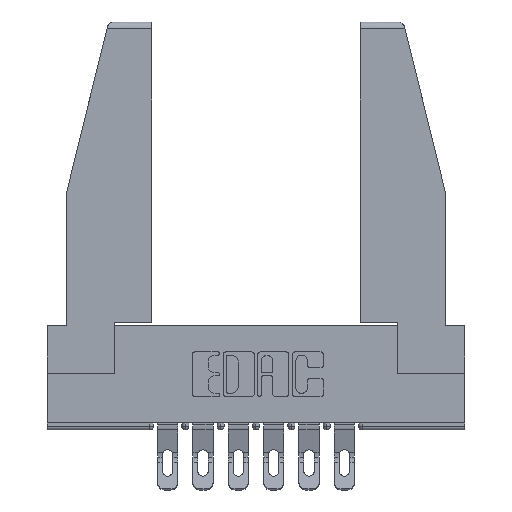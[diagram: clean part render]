
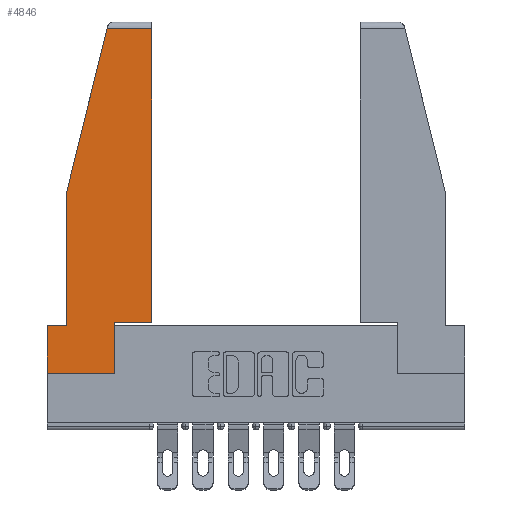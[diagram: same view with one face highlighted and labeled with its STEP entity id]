
A CAD part, top view. The second image highlights one B-rep face of the part: STEP entity #4846.
In plain terms, the highlighted planar face has unit normal (0, 0, 1).
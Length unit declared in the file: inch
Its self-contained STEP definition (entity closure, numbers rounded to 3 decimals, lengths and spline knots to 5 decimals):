
#361 = EDGE_CURVE ( 'NONE', #10906, #6399, #10309, .T. ) ;
#398 = CARTESIAN_POINT ( 'NONE',  ( 0.297, 0.223, 0. ) ) ;
#401 = EDGE_CURVE ( 'NONE', #5165, #10906, #4209, .T. ) ;
#894 = VERTEX_POINT ( 'NONE', #1363 ) ;
#895 = ORIENTED_EDGE ( 'NONE', *, *, #5038, .T. ) ;
#1025 = VECTOR ( 'NONE', #11948, 39.37008 ) ;
#1055 = VECTOR ( 'NONE', #4365, 39.37008 ) ;
#1147 = LINE ( 'NONE', #11577, #8379 ) ;
#1281 = ORIENTED_EDGE ( 'NONE', *, *, #6685, .T. ) ;
#1363 = CARTESIAN_POINT ( 'NONE',  ( 0.461, 0.223, 0. ) ) ;
#1478 = CARTESIAN_POINT ( 'NONE',  ( 0., 0., 0. ) ) ;
#1511 = CARTESIAN_POINT ( 'NONE',  ( 0.461, 0.223, 0. ) ) ;
#1646 = VECTOR ( 'NONE', #2559, 39.37008 ) ;
#1691 = ORIENTED_EDGE ( 'NONE', *, *, #6602, .T. ) ;
#1863 = CARTESIAN_POINT ( 'NONE',  ( 0., 0.21, 0. ) ) ;
#2161 = CARTESIAN_POINT ( 'NONE',  ( 0.461, 1.52, 0. ) ) ;
#2559 = DIRECTION ( 'NONE',  ( 1., 0., 0. ) ) ;
#2609 = EDGE_LOOP ( 'NONE', ( #10805, #1281, #4239, #11227, #1691, #8026, #3863, #895, #3828 ) ) ;
#2720 = CARTESIAN_POINT ( 'NONE',  ( 0.2636, 1.52, 0. ) ) ;
#2791 = EDGE_CURVE ( 'NONE', #12323, #894, #1147, .T. ) ;
#3111 = VERTEX_POINT ( 'NONE', #9955 ) ;
#3147 = LINE ( 'NONE', #1511, #10051 ) ;
#3241 = CARTESIAN_POINT ( 'NONE',  ( 0.086, 0.8, 0. ) ) ;
#3828 = ORIENTED_EDGE ( 'NONE', *, *, #2791, .T. ) ;
#3863 = ORIENTED_EDGE ( 'NONE', *, *, #10009, .T. ) ;
#3896 = VECTOR ( 'NONE', #6126, 39.37008 ) ;
#3951 = LINE ( 'NONE', #8561, #6805 ) ;
#4178 = EDGE_CURVE ( 'NONE', #4179, #9728, #4284, .T. ) ;
#4179 = VERTEX_POINT ( 'NONE', #6166 ) ;
#4209 = LINE ( 'NONE', #7589, #1025 ) ;
#4239 = ORIENTED_EDGE ( 'NONE', *, *, #401, .T. ) ;
#4284 = LINE ( 'NONE', #1863, #13579 ) ;
#4365 = DIRECTION ( 'NONE',  ( -1., 0., 0. ) ) ;
#4571 = LINE ( 'NONE', #8563, #1055 ) ;
#4846 = ADVANCED_FACE ( 'NONE', ( #12068 ), #12725, .T. ) ;
#5038 = EDGE_CURVE ( 'NONE', #3111, #12323, #3951, .T. ) ;
#5055 = CARTESIAN_POINT ( 'NONE',  ( 0.086, 0.8, 0. ) ) ;
#5165 = VERTEX_POINT ( 'NONE', #2720 ) ;
#5220 = CARTESIAN_POINT ( 'NONE',  ( 0., 0., 0. ) ) ;
#5256 = CARTESIAN_POINT ( 'NONE',  ( 0., 0., 0. ) ) ;
#6126 = DIRECTION ( 'NONE',  ( 0., -1., 0. ) ) ;
#6166 = CARTESIAN_POINT ( 'NONE',  ( 0., 0.21, 0. ) ) ;
#6399 = VERTEX_POINT ( 'NONE', #10354 ) ;
#6602 = EDGE_CURVE ( 'NONE', #6399, #4179, #12688, .T. ) ;
#6685 = EDGE_CURVE ( 'NONE', #13383, #5165, #4571, .T. ) ;
#6710 = AXIS2_PLACEMENT_3D ( 'NONE', #5256, #8372, #13804 ) ;
#6805 = VECTOR ( 'NONE', #8607, 39.37008 ) ;
#7589 = CARTESIAN_POINT ( 'NONE',  ( 0.271, 1.55, 0. ) ) ;
#8026 = ORIENTED_EDGE ( 'NONE', *, *, #4178, .T. ) ;
#8372 = DIRECTION ( 'NONE',  ( 0., 0., 1. ) ) ;
#8379 = VECTOR ( 'NONE', #13820, 39.37008 ) ;
#8561 = CARTESIAN_POINT ( 'NONE',  ( 0.297, 0., 0. ) ) ;
#8563 = CARTESIAN_POINT ( 'NONE',  ( 0., 1.52, 0. ) ) ;
#8607 = DIRECTION ( 'NONE',  ( 0., 1., 0. ) ) ;
#9029 = DIRECTION ( 'NONE',  ( 0., 1., 0. ) ) ;
#9410 = DIRECTION ( 'NONE',  ( -1., 0., 0. ) ) ;
#9685 = DIRECTION ( 'NONE',  ( 0., -1., 0. ) ) ;
#9728 = VERTEX_POINT ( 'NONE', #5220 ) ;
#9822 = VECTOR ( 'NONE', #9410, 39.37008 ) ;
#9955 = CARTESIAN_POINT ( 'NONE',  ( 0.297, 0., 0. ) ) ;
#10009 = EDGE_CURVE ( 'NONE', #9728, #3111, #10752, .T. ) ;
#10051 = VECTOR ( 'NONE', #9029, 39.37008 ) ;
#10309 = LINE ( 'NONE', #5055, #3896 ) ;
#10354 = CARTESIAN_POINT ( 'NONE',  ( 0.086, 0.21, 0. ) ) ;
#10543 = EDGE_CURVE ( 'NONE', #894, #13383, #3147, .T. ) ;
#10752 = LINE ( 'NONE', #1478, #1646 ) ;
#10805 = ORIENTED_EDGE ( 'NONE', *, *, #10543, .T. ) ;
#10906 = VERTEX_POINT ( 'NONE', #3241 ) ;
#11227 = ORIENTED_EDGE ( 'NONE', *, *, #361, .T. ) ;
#11577 = CARTESIAN_POINT ( 'NONE',  ( 0.297, 0.223, 0. ) ) ;
#11653 = CARTESIAN_POINT ( 'NONE',  ( 0., 0.21, 0. ) ) ;
#11948 = DIRECTION ( 'NONE',  ( -0.239, -0.971, 0. ) ) ;
#12068 = FACE_OUTER_BOUND ( 'NONE', #2609, .T. ) ;
#12323 = VERTEX_POINT ( 'NONE', #398 ) ;
#12688 = LINE ( 'NONE', #11653, #9822 ) ;
#12725 = PLANE ( 'NONE',  #6710 ) ;
#13383 = VERTEX_POINT ( 'NONE', #2161 ) ;
#13579 = VECTOR ( 'NONE', #9685, 39.37008 ) ;
#13804 = DIRECTION ( 'NONE',  ( 1., 0., 0. ) ) ;
#13820 = DIRECTION ( 'NONE',  ( 1., 0., 0. ) ) ;
